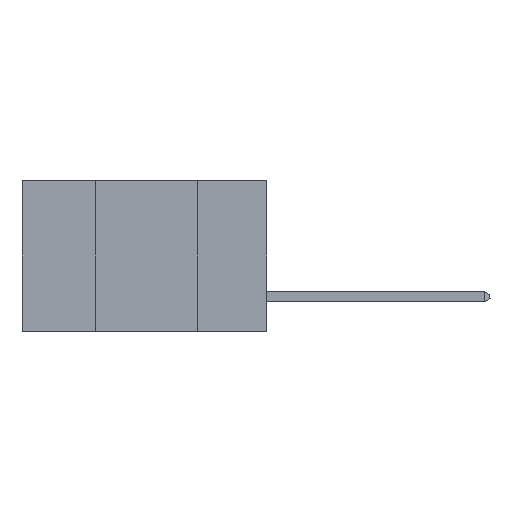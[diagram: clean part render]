
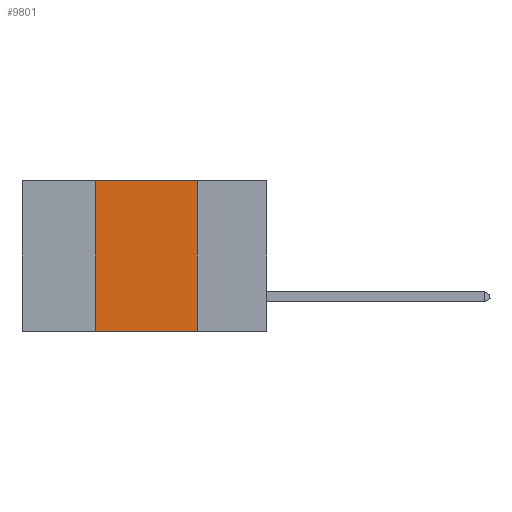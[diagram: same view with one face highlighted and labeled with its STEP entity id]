
A CAD part, left-side view. The second image highlights one B-rep face of the part: STEP entity #9801.
In plain terms, the highlighted planar face has unit normal (-1, 0, 0).
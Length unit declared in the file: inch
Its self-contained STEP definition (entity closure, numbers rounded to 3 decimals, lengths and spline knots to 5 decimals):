
#420 = DIRECTION ( 'NONE',  ( 0., 0., -1. ) ) ;
#598 = VECTOR ( 'NONE', #11464, 39.37008 ) ;
#1423 = FACE_OUTER_BOUND ( 'NONE', #9741, .T. ) ;
#2113 = VECTOR ( 'NONE', #3768, 39.37008 ) ;
#2564 = AXIS2_PLACEMENT_3D ( 'NONE', #14565, #12926, #420 ) ;
#3404 = ORIENTED_EDGE ( 'NONE', *, *, #12077, .T. ) ;
#3645 = PLANE ( 'NONE',  #2564 ) ;
#3749 = ORIENTED_EDGE ( 'NONE', *, *, #10650, .F. ) ;
#3768 = DIRECTION ( 'NONE',  ( 0., 0., 1. ) ) ;
#4445 = VERTEX_POINT ( 'NONE', #16411 ) ;
#5388 = ORIENTED_EDGE ( 'NONE', *, *, #7039, .F. ) ;
#5431 = ORIENTED_EDGE ( 'NONE', *, *, #11265, .F. ) ;
#5577 = CARTESIAN_POINT ( 'NONE',  ( 0., 0.6, -0.37 ) ) ;
#6179 = CARTESIAN_POINT ( 'NONE',  ( 0., 0.42, -0.37 ) ) ;
#6502 = VERTEX_POINT ( 'NONE', #12886 ) ;
#6704 = LINE ( 'NONE', #12975, #2113 ) ;
#6795 = DIRECTION ( 'NONE',  ( 0., 0., -1. ) ) ;
#6846 = VECTOR ( 'NONE', #13367, 39.37008 ) ;
#7039 = EDGE_CURVE ( 'NONE', #4445, #6502, #10722, .T. ) ;
#7322 = VERTEX_POINT ( 'NONE', #6179 ) ;
#9741 = EDGE_LOOP ( 'NONE', ( #5431, #5388, #3749, #3404 ) ) ;
#9801 = ADVANCED_FACE ( 'NONE', ( #1423 ), #3645, .F. ) ;
#10002 = LINE ( 'NONE', #17637, #11480 ) ;
#10028 = CARTESIAN_POINT ( 'NONE',  ( 0., 0.17, -0.37 ) ) ;
#10650 = EDGE_CURVE ( 'NONE', #7322, #4445, #6704, .T. ) ;
#10722 = LINE ( 'NONE', #19117, #598 ) ;
#11265 = EDGE_CURVE ( 'NONE', #6502, #18646, #10002, .T. ) ;
#11464 = DIRECTION ( 'NONE',  ( 0., -1., 0. ) ) ;
#11480 = VECTOR ( 'NONE', #6795, 39.37008 ) ;
#12077 = EDGE_CURVE ( 'NONE', #7322, #18646, #14356, .T. ) ;
#12886 = CARTESIAN_POINT ( 'NONE',  ( 0., 0.17, 0. ) ) ;
#12926 = DIRECTION ( 'NONE',  ( 1., 0., 0. ) ) ;
#12975 = CARTESIAN_POINT ( 'NONE',  ( 0., 0.42, 0. ) ) ;
#13367 = DIRECTION ( 'NONE',  ( 0., -1., 0. ) ) ;
#14356 = LINE ( 'NONE', #5577, #6846 ) ;
#14565 = CARTESIAN_POINT ( 'NONE',  ( 0., 0.6, 0. ) ) ;
#16411 = CARTESIAN_POINT ( 'NONE',  ( 0., 0.42, 0. ) ) ;
#17637 = CARTESIAN_POINT ( 'NONE',  ( 0., 0.17, 0. ) ) ;
#18646 = VERTEX_POINT ( 'NONE', #10028 ) ;
#19117 = CARTESIAN_POINT ( 'NONE',  ( 0., 0.6, 0. ) ) ;
